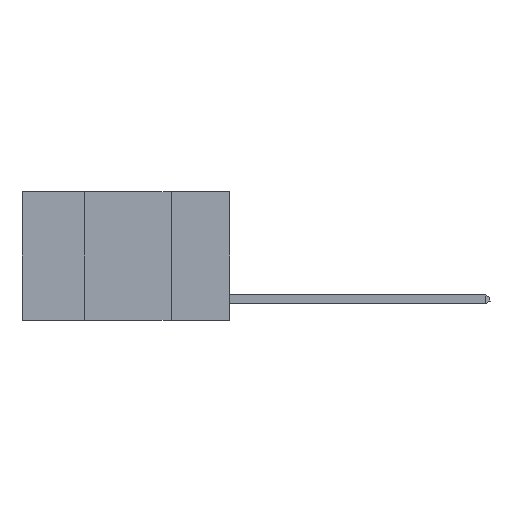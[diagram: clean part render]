
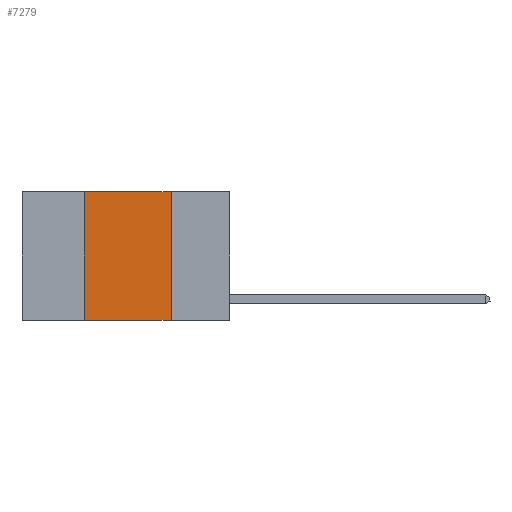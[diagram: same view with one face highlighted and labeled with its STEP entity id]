
A CAD part, left-side view. The second image highlights one B-rep face of the part: STEP entity #7279.
In plain terms, the highlighted planar face has unit normal (-1, 0, 0).
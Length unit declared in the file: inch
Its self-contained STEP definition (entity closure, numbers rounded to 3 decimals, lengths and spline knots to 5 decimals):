
#852 = VECTOR ( 'NONE', #8897, 39.37008 ) ;
#986 = EDGE_CURVE ( 'NONE', #13849, #11597, #9125, .T. ) ;
#1086 = VECTOR ( 'NONE', #10186, 39.37008 ) ;
#1407 = FACE_OUTER_BOUND ( 'NONE', #7698, .T. ) ;
#1620 = ORIENTED_EDGE ( 'NONE', *, *, #15603, .F. ) ;
#2325 = LINE ( 'NONE', #12108, #16648 ) ;
#3224 = LINE ( 'NONE', #15859, #852 ) ;
#4255 = CARTESIAN_POINT ( 'NONE',  ( 0., 0.17, 0. ) ) ;
#5084 = ORIENTED_EDGE ( 'NONE', *, *, #986, .T. ) ;
#5746 = EDGE_CURVE ( 'NONE', #13849, #6503, #9159, .T. ) ;
#6503 = VERTEX_POINT ( 'NONE', #17009 ) ;
#7279 = ADVANCED_FACE ( 'NONE', ( #1407 ), #12942, .F. ) ;
#7646 = DIRECTION ( 'NONE',  ( 0., -1., 0. ) ) ;
#7698 = EDGE_LOOP ( 'NONE', ( #12728, #1620, #14639, #5084 ) ) ;
#8458 = CARTESIAN_POINT ( 'NONE',  ( 0., 0.42, -0.37 ) ) ;
#8897 = DIRECTION ( 'NONE',  ( 0., -1., 0. ) ) ;
#9125 = LINE ( 'NONE', #11532, #18354 ) ;
#9159 = LINE ( 'NONE', #11957, #1086 ) ;
#10078 = DIRECTION ( 'NONE',  ( 1., 0., 0. ) ) ;
#10186 = DIRECTION ( 'NONE',  ( 0., 0., 1. ) ) ;
#11532 = CARTESIAN_POINT ( 'NONE',  ( 0., 0.6, -0.37 ) ) ;
#11597 = VERTEX_POINT ( 'NONE', #15207 ) ;
#11957 = CARTESIAN_POINT ( 'NONE',  ( 0., 0.42, 0. ) ) ;
#12108 = CARTESIAN_POINT ( 'NONE',  ( 0., 0.17, 0. ) ) ;
#12728 = ORIENTED_EDGE ( 'NONE', *, *, #17540, .F. ) ;
#12942 = PLANE ( 'NONE',  #18128 ) ;
#13849 = VERTEX_POINT ( 'NONE', #8458 ) ;
#13923 = VERTEX_POINT ( 'NONE', #4255 ) ;
#14332 = CARTESIAN_POINT ( 'NONE',  ( 0., 0.6, 0. ) ) ;
#14639 = ORIENTED_EDGE ( 'NONE', *, *, #5746, .F. ) ;
#15207 = CARTESIAN_POINT ( 'NONE',  ( 0., 0.17, -0.37 ) ) ;
#15603 = EDGE_CURVE ( 'NONE', #6503, #13923, #3224, .T. ) ;
#15726 = DIRECTION ( 'NONE',  ( 0., 0., -1. ) ) ;
#15859 = CARTESIAN_POINT ( 'NONE',  ( 0., 0.6, 0. ) ) ;
#16091 = DIRECTION ( 'NONE',  ( 0., 0., -1. ) ) ;
#16648 = VECTOR ( 'NONE', #16091, 39.37008 ) ;
#17009 = CARTESIAN_POINT ( 'NONE',  ( 0., 0.42, 0. ) ) ;
#17540 = EDGE_CURVE ( 'NONE', #13923, #11597, #2325, .T. ) ;
#18128 = AXIS2_PLACEMENT_3D ( 'NONE', #14332, #10078, #15726 ) ;
#18354 = VECTOR ( 'NONE', #7646, 39.37008 ) ;
